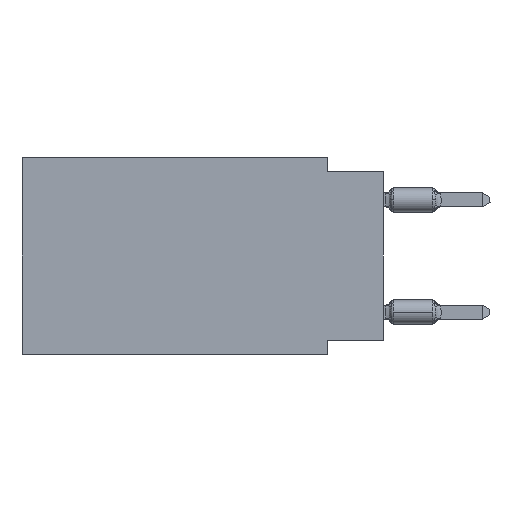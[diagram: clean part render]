
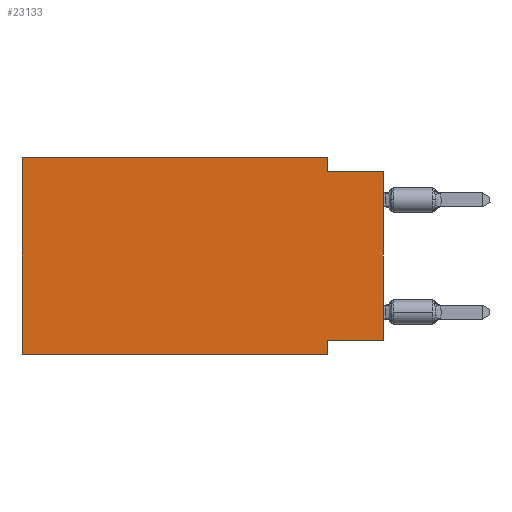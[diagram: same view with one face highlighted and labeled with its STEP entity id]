
A CAD part, left-side view. The second image highlights one B-rep face of the part: STEP entity #23133.
In plain terms, the highlighted planar face has unit normal (-1, 0, 0).
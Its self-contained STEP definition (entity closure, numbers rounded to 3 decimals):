
#203 = DIRECTION ( 'NONE',  ( 0., 0., -1. ) ) ;
#1000 = EDGE_CURVE ( 'NONE', #17261, #24502, #32020, .T. ) ;
#1861 = VECTOR ( 'NONE', #15390, 1000. ) ;
#2285 = DIRECTION ( 'NONE',  ( 0., 0., -1. ) ) ;
#2363 = DIRECTION ( 'NONE',  ( 0., 0., 1. ) ) ;
#2400 = DIRECTION ( 'NONE',  ( 0., -1., 0. ) ) ;
#2633 = ORIENTED_EDGE ( 'NONE', *, *, #19404, .F. ) ;
#2954 = VERTEX_POINT ( 'NONE', #35179 ) ;
#5374 = LINE ( 'NONE', #32857, #20396 ) ;
#7663 = EDGE_LOOP ( 'NONE', ( #23438, #29146, #17665, #29045, #16048, #8781, #2633, #21057 ) ) ;
#8008 = CARTESIAN_POINT ( 'NONE',  ( 0., 0., -0.635 ) ) ;
#8280 = DIRECTION ( 'NONE',  ( 0., 1., 0. ) ) ;
#8415 = VECTOR ( 'NONE', #2400, 1000. ) ;
#8536 = LINE ( 'NONE', #27704, #9542 ) ;
#8781 = ORIENTED_EDGE ( 'NONE', *, *, #31410, .T. ) ;
#9542 = VECTOR ( 'NONE', #203, 1000. ) ;
#9747 = CARTESIAN_POINT ( 'NONE',  ( 0., 16.383, 0. ) ) ;
#9953 = CARTESIAN_POINT ( 'NONE',  ( 0., 16.383, 0. ) ) ;
#10262 = CARTESIAN_POINT ( 'NONE',  ( 0., 2.54, -8.89 ) ) ;
#10498 = LINE ( 'NONE', #18445, #1861 ) ;
#13146 = EDGE_CURVE ( 'NONE', #21335, #25690, #27171, .T. ) ;
#13976 = AXIS2_PLACEMENT_3D ( 'NONE', #9953, #34889, #31825 ) ;
#14357 = CARTESIAN_POINT ( 'NONE',  ( 0., 2.54, 0. ) ) ;
#15275 = EDGE_CURVE ( 'NONE', #32467, #2954, #5374, .T. ) ;
#15390 = DIRECTION ( 'NONE',  ( 0., 0., 1. ) ) ;
#15560 = FACE_OUTER_BOUND ( 'NONE', #7663, .T. ) ;
#15750 = CARTESIAN_POINT ( 'NONE',  ( 0., 16.383, 0. ) ) ;
#16048 = ORIENTED_EDGE ( 'NONE', *, *, #1000, .F. ) ;
#16098 = PLANE ( 'NONE',  #13976 ) ;
#16301 = VECTOR ( 'NONE', #2285, 1000. ) ;
#16460 = CARTESIAN_POINT ( 'NONE',  ( 0., 2.54, -8.89 ) ) ;
#16597 = VERTEX_POINT ( 'NONE', #14357 ) ;
#16880 = EDGE_CURVE ( 'NONE', #16597, #21335, #8536, .T. ) ;
#17261 = VERTEX_POINT ( 'NONE', #27662 ) ;
#17271 = VERTEX_POINT ( 'NONE', #16460 ) ;
#17665 = ORIENTED_EDGE ( 'NONE', *, *, #16880, .F. ) ;
#18445 = CARTESIAN_POINT ( 'NONE',  ( 0., 0., 0. ) ) ;
#19053 = CARTESIAN_POINT ( 'NONE',  ( 0., 2.54, -0.635 ) ) ;
#19404 = EDGE_CURVE ( 'NONE', #2954, #17271, #29953, .T. ) ;
#19434 = VECTOR ( 'NONE', #24447, 1000. ) ;
#20260 = LINE ( 'NONE', #25514, #20588 ) ;
#20396 = VECTOR ( 'NONE', #8280, 1000. ) ;
#20588 = VECTOR ( 'NONE', #31313, 1000. ) ;
#21057 = ORIENTED_EDGE ( 'NONE', *, *, #15275, .F. ) ;
#21335 = VERTEX_POINT ( 'NONE', #19053 ) ;
#23099 = EDGE_CURVE ( 'NONE', #32467, #25690, #10498, .T. ) ;
#23133 = ADVANCED_FACE ( 'NONE', ( #15560 ), #16098, .F. ) ;
#23438 = ORIENTED_EDGE ( 'NONE', *, *, #23099, .T. ) ;
#24447 = DIRECTION ( 'NONE',  ( 0., -1., 0. ) ) ;
#24502 = VERTEX_POINT ( 'NONE', #9747 ) ;
#24534 = VECTOR ( 'NONE', #2363, 1000. ) ;
#25514 = CARTESIAN_POINT ( 'NONE',  ( 0., 16.383, -8.89 ) ) ;
#25690 = VERTEX_POINT ( 'NONE', #29630 ) ;
#26671 = EDGE_CURVE ( 'NONE', #24502, #16597, #35665, .T. ) ;
#27171 = LINE ( 'NONE', #8008, #8415 ) ;
#27662 = CARTESIAN_POINT ( 'NONE',  ( 0., 16.383, -8.89 ) ) ;
#27704 = CARTESIAN_POINT ( 'NONE',  ( 0., 2.54, 0. ) ) ;
#29045 = ORIENTED_EDGE ( 'NONE', *, *, #26671, .F. ) ;
#29146 = ORIENTED_EDGE ( 'NONE', *, *, #13146, .F. ) ;
#29630 = CARTESIAN_POINT ( 'NONE',  ( 0., 0., -0.635 ) ) ;
#29953 = LINE ( 'NONE', #10262, #16301 ) ;
#30247 = CARTESIAN_POINT ( 'NONE',  ( 0., 16.383, 0. ) ) ;
#31313 = DIRECTION ( 'NONE',  ( 0., -1., 0. ) ) ;
#31410 = EDGE_CURVE ( 'NONE', #17261, #17271, #20260, .T. ) ;
#31825 = DIRECTION ( 'NONE',  ( 0., 0., -1. ) ) ;
#32020 = LINE ( 'NONE', #15750, #24534 ) ;
#32467 = VERTEX_POINT ( 'NONE', #35668 ) ;
#32857 = CARTESIAN_POINT ( 'NONE',  ( 0., 0., -8.255 ) ) ;
#34889 = DIRECTION ( 'NONE',  ( 1., 0., 0. ) ) ;
#35179 = CARTESIAN_POINT ( 'NONE',  ( 0., 2.54, -8.255 ) ) ;
#35665 = LINE ( 'NONE', #30247, #19434 ) ;
#35668 = CARTESIAN_POINT ( 'NONE',  ( 0., 0., -8.255 ) ) ;
